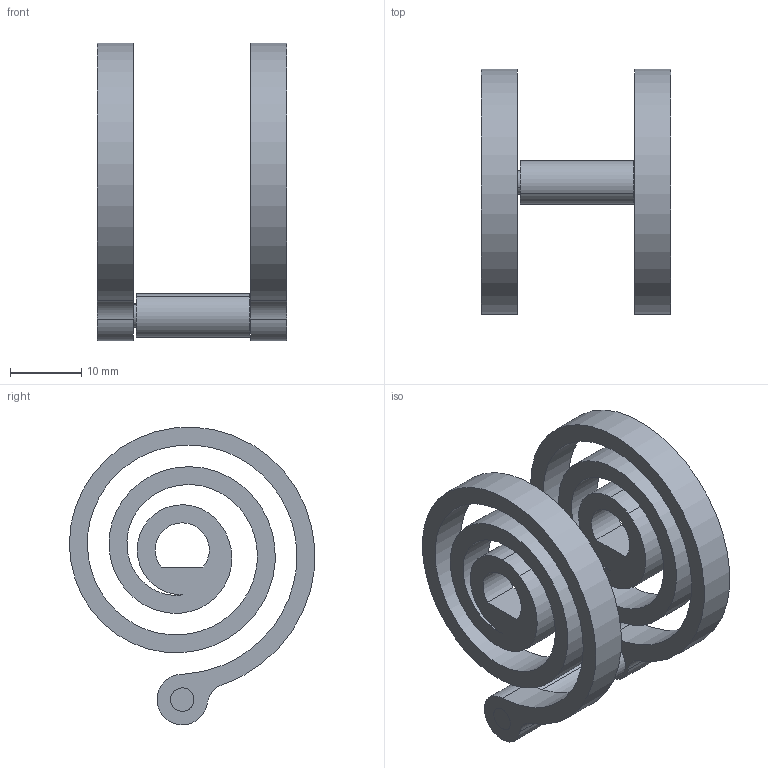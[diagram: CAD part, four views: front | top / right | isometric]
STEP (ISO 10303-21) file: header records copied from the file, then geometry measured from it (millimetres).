
FILE_DESCRIPTION (( 'STEP AP214' ), '1' );
FILE_NAME ('HammerSpringAssem.STEP', '2013-06-07T17:14:29', ( 'Asher' ), ( '' ), 'SwSTEP 2.0', 'SolidWorks 2013', '' );
FILE_SCHEMA (( 'AUTOMOTIVE_DESIGN' ));
Length unit declared in the file: inch
Products named in the file (4): HammerSpringAssem; Spring; spring_connecting_rod_bushing; spring_connecting_rod
Assembly tree (4 placements, depth 2):
  HammerSpringAssem
    Spring  x2
    spring_connecting_rod_bushing
    spring_connecting_rod
Bounding box: 26.67 x 34.54 x 41.89 mm (x, y, z)
Volume: 6111.3 mm3; surface area: 7347.3 mm2
Topology: 4 solids, 4 shells, 38 faces, 90 edges, 60 vertices
Faces by surface type: cylinder 22, plane 10, bspline 6
Entity records: 1346 total; most frequent: CARTESIAN_POINT 608, DIRECTION 132, ORIENTED_EDGE 108, AXIS2_PLACEMENT_3D 56, EDGE_CURVE 54, VERTEX_POINT 36, EDGE_LOOP 30, CIRCLE 28
